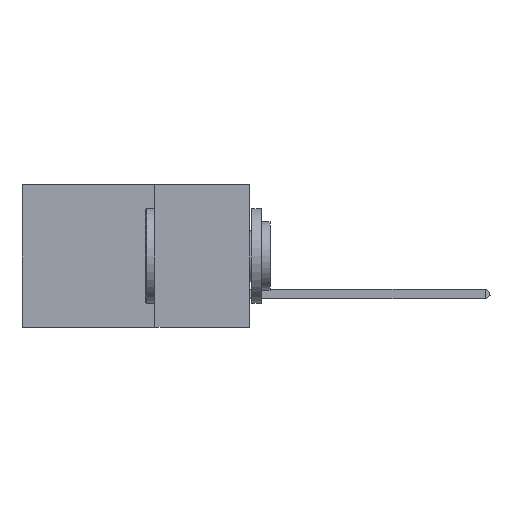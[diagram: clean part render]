
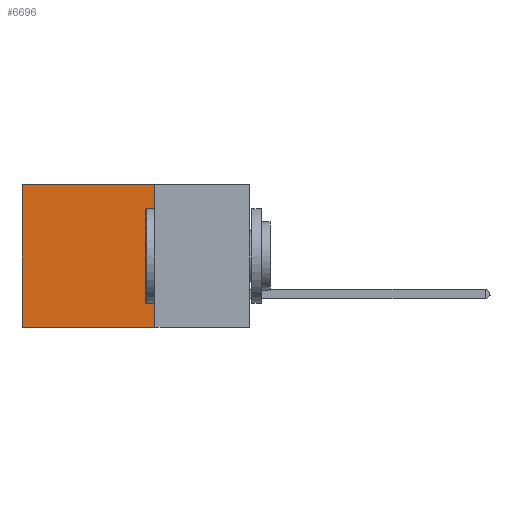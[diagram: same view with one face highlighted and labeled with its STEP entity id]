
A CAD part, left-side view. The second image highlights one B-rep face of the part: STEP entity #6696.
In plain terms, the highlighted planar face has unit normal (-1, 0, 0).
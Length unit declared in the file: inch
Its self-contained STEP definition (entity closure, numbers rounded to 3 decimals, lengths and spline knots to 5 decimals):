
#67 = ORIENTED_EDGE ( 'NONE', *, *, #8554, .T. ) ;
#426 = EDGE_CURVE ( 'NONE', #2834, #11155, #15562, .T. ) ;
#1910 = CARTESIAN_POINT ( 'NONE',  ( 0.2875, 0.25, 0. ) ) ;
#2489 = VECTOR ( 'NONE', #12497, 39.37008 ) ;
#2513 = EDGE_CURVE ( 'NONE', #7266, #11940, #7417, .T. ) ;
#2778 = CARTESIAN_POINT ( 'NONE',  ( 0.2875, 0.6, -0.375 ) ) ;
#2834 = VERTEX_POINT ( 'NONE', #7179 ) ;
#3139 = FACE_OUTER_BOUND ( 'NONE', #10710, .T. ) ;
#3628 = DIRECTION ( 'NONE',  ( 0., 0., -1. ) ) ;
#4338 = DIRECTION ( 'NONE',  ( 0., 0., -1. ) ) ;
#4962 = ORIENTED_EDGE ( 'NONE', *, *, #426, .T. ) ;
#5043 = PLANE ( 'NONE',  #6469 ) ;
#5056 = LINE ( 'NONE', #8566, #10745 ) ;
#5520 = VECTOR ( 'NONE', #4338, 39.37008 ) ;
#6433 = VECTOR ( 'NONE', #10449, 39.37008 ) ;
#6469 = AXIS2_PLACEMENT_3D ( 'NONE', #12305, #9815, #3628 ) ;
#6547 = CARTESIAN_POINT ( 'NONE',  ( 0.2875, 0.25, -0.375 ) ) ;
#6696 = ADVANCED_FACE ( 'NONE', ( #3139 ), #5043, .F. ) ;
#6796 = EDGE_CURVE ( 'NONE', #2834, #7266, #5056, .T. ) ;
#7179 = CARTESIAN_POINT ( 'NONE',  ( 0.2875, 0.25, 0. ) ) ;
#7266 = VERTEX_POINT ( 'NONE', #14533 ) ;
#7417 = LINE ( 'NONE', #6547, #2489 ) ;
#8554 = EDGE_CURVE ( 'NONE', #11155, #11940, #12725, .T. ) ;
#8566 = CARTESIAN_POINT ( 'NONE',  ( 0.2875, 0.25, -0.375 ) ) ;
#9755 = ORIENTED_EDGE ( 'NONE', *, *, #2513, .F. ) ;
#9815 = DIRECTION ( 'NONE',  ( 1., 0., 0. ) ) ;
#10195 = CARTESIAN_POINT ( 'NONE',  ( 0.2875, 0.6, -0.375 ) ) ;
#10449 = DIRECTION ( 'NONE',  ( 0., 1., 0. ) ) ;
#10710 = EDGE_LOOP ( 'NONE', ( #67, #9755, #14177, #4962 ) ) ;
#10745 = VECTOR ( 'NONE', #13477, 39.37008 ) ;
#11155 = VERTEX_POINT ( 'NONE', #11407 ) ;
#11407 = CARTESIAN_POINT ( 'NONE',  ( 0.2875, 0.6, 0. ) ) ;
#11940 = VERTEX_POINT ( 'NONE', #2778 ) ;
#12305 = CARTESIAN_POINT ( 'NONE',  ( 0.2875, 0.25, -0.375 ) ) ;
#12497 = DIRECTION ( 'NONE',  ( 0., 1., 0. ) ) ;
#12725 = LINE ( 'NONE', #10195, #5520 ) ;
#13477 = DIRECTION ( 'NONE',  ( 0., 0., -1. ) ) ;
#14177 = ORIENTED_EDGE ( 'NONE', *, *, #6796, .F. ) ;
#14533 = CARTESIAN_POINT ( 'NONE',  ( 0.2875, 0.25, -0.375 ) ) ;
#15562 = LINE ( 'NONE', #1910, #6433 ) ;
